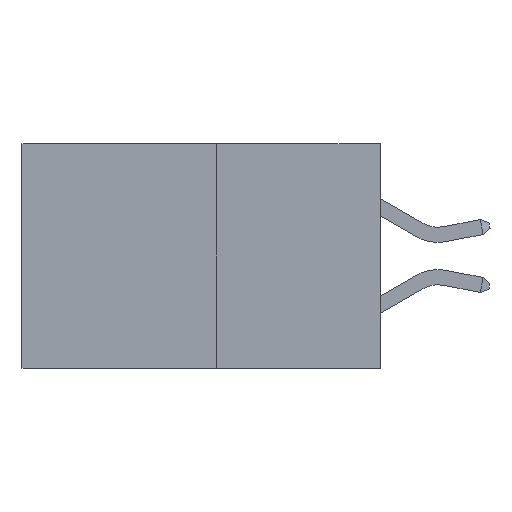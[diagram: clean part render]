
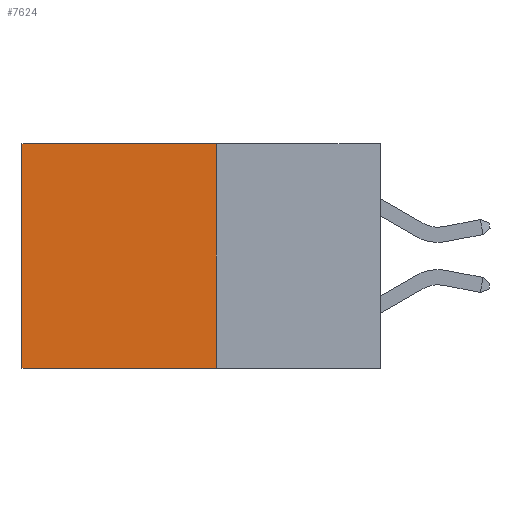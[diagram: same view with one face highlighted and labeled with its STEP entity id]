
A CAD part, left-side view. The second image highlights one B-rep face of the part: STEP entity #7624.
In plain terms, the highlighted planar face has unit normal (-1, 0, 0).
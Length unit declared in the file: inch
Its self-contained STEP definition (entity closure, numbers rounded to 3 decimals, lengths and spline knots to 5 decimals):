
#158 = CARTESIAN_POINT ( 'NONE',  ( 0.277, 0.27, -0.37 ) ) ;
#292 = DIRECTION ( 'NONE',  ( 0., 0., -1. ) ) ;
#303 = CARTESIAN_POINT ( 'NONE',  ( 0.277, 0.27, 0. ) ) ;
#658 = ORIENTED_EDGE ( 'NONE', *, *, #1528, .F. ) ;
#811 = CARTESIAN_POINT ( 'NONE',  ( 0.277, 0.27, 0. ) ) ;
#927 = CARTESIAN_POINT ( 'NONE',  ( 0.277, 0.59, -0.37 ) ) ;
#970 = LINE ( 'NONE', #4556, #7757 ) ;
#1139 = LINE ( 'NONE', #4270, #4561 ) ;
#1528 = EDGE_CURVE ( 'NONE', #6519, #2541, #970, .T. ) ;
#1562 = ORIENTED_EDGE ( 'NONE', *, *, #6654, .F. ) ;
#2148 = DIRECTION ( 'NONE',  ( 0., 0., -1. ) ) ;
#2181 = EDGE_CURVE ( 'NONE', #4797, #4907, #4901, .T. ) ;
#2228 = EDGE_LOOP ( 'NONE', ( #2414, #658, #1562, #8296 ) ) ;
#2235 = CARTESIAN_POINT ( 'NONE',  ( 0.277, 0.27, -0.37 ) ) ;
#2414 = ORIENTED_EDGE ( 'NONE', *, *, #3520, .T. ) ;
#2541 = VERTEX_POINT ( 'NONE', #927 ) ;
#3520 = EDGE_CURVE ( 'NONE', #4907, #2541, #1139, .T. ) ;
#3872 = VECTOR ( 'NONE', #292, 39.37008 ) ;
#4086 = LINE ( 'NONE', #158, #3872 ) ;
#4111 = FACE_OUTER_BOUND ( 'NONE', #2228, .T. ) ;
#4270 = CARTESIAN_POINT ( 'NONE',  ( 0.277, 0.59, -0.37 ) ) ;
#4556 = CARTESIAN_POINT ( 'NONE',  ( 0.277, 0.27, -0.37 ) ) ;
#4561 = VECTOR ( 'NONE', #2148, 39.37008 ) ;
#4703 = DIRECTION ( 'NONE',  ( 0., 1., 0. ) ) ;
#4797 = VERTEX_POINT ( 'NONE', #303 ) ;
#4901 = LINE ( 'NONE', #811, #6707 ) ;
#4907 = VERTEX_POINT ( 'NONE', #7897 ) ;
#5278 = AXIS2_PLACEMENT_3D ( 'NONE', #6236, #6208, #6199 ) ;
#6199 = DIRECTION ( 'NONE',  ( 0., 0., -1. ) ) ;
#6208 = DIRECTION ( 'NONE',  ( 1., 0., 0. ) ) ;
#6236 = CARTESIAN_POINT ( 'NONE',  ( 0.277, 0.27, -0.37 ) ) ;
#6256 = PLANE ( 'NONE',  #5278 ) ;
#6519 = VERTEX_POINT ( 'NONE', #2235 ) ;
#6654 = EDGE_CURVE ( 'NONE', #4797, #6519, #4086, .T. ) ;
#6707 = VECTOR ( 'NONE', #8063, 39.37008 ) ;
#7624 = ADVANCED_FACE ( 'NONE', ( #4111 ), #6256, .F. ) ;
#7757 = VECTOR ( 'NONE', #4703, 39.37008 ) ;
#7897 = CARTESIAN_POINT ( 'NONE',  ( 0.277, 0.59, 0. ) ) ;
#8063 = DIRECTION ( 'NONE',  ( 0., 1., 0. ) ) ;
#8296 = ORIENTED_EDGE ( 'NONE', *, *, #2181, .T. ) ;
